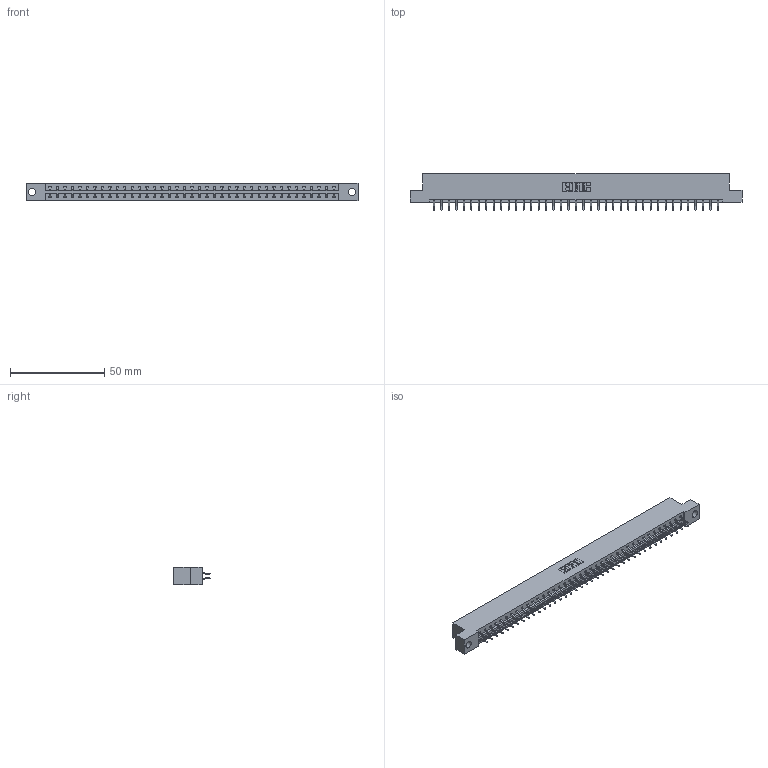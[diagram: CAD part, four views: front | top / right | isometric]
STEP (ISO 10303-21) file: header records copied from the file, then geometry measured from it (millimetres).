
FILE_DESCRIPTION (( 'STEP AP203' ), '1' );
FILE_NAME ('833-078-556-204.STEP', '2020-06-05T20:36:28', ( '' ), ( '' ), 'SwSTEP 2.0', 'SolidWorks 2020', '' );
FILE_SCHEMA (( 'CONFIG_CONTROL_DESIGN' ));
Length unit declared in the file: inch
Products named in the file (3): 833-078-556-204; 345-292-001_556 Tail; 833 Part_Flush - .156 Dia - TH
Assembly tree (79 placements, depth 2):
  833-078-556-204
    833 Part_Flush - .156 Dia - TH
    345-292-001_556 Tail  x78
Bounding box: 176.07 x 19.57 x 9.4 mm (x, y, z)
Volume: 17857 mm3; surface area: 20801.7 mm2
Topology: 79 solids, 79 shells, 4638 faces, 13805 edges, 9098 vertices
Faces by surface type: plane 3190, cylinder 1448
Entity records: 25701 total; most frequent: CARTESIAN_POINT 4278, ORIENTED_EDGE 4202, DIRECTION 3649, EDGE_CURVE 2101, LINE 1965, VECTOR 1965, VERTEX_POINT 1398, AXIS2_PLACEMENT_3D 842
